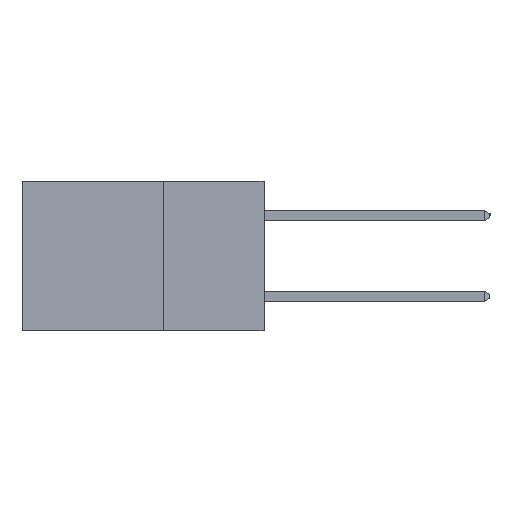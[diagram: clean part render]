
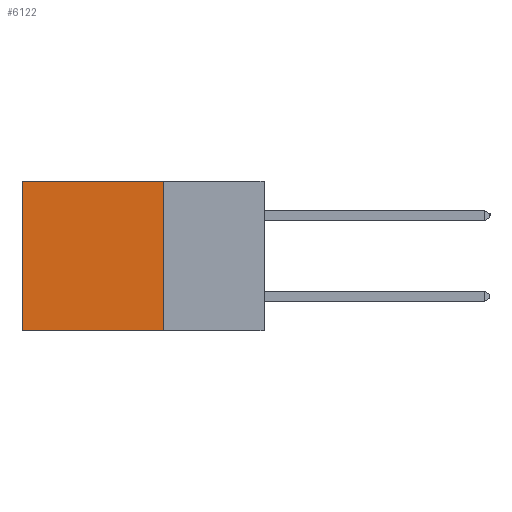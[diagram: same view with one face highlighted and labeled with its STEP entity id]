
A CAD part, left-side view. The second image highlights one B-rep face of the part: STEP entity #6122.
In plain terms, the highlighted planar face has unit normal (-1, 0, 0).
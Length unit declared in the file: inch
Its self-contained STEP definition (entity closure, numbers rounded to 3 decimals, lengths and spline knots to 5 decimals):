
#562 = AXIS2_PLACEMENT_3D ( 'NONE', #2618, #17270, #15629 ) ;
#961 = ORIENTED_EDGE ( 'NONE', *, *, #13653, .T. ) ;
#1107 = CARTESIAN_POINT ( 'NONE',  ( 0.2615, 0.6, -0.37 ) ) ;
#2184 = ORIENTED_EDGE ( 'NONE', *, *, #2893, .F. ) ;
#2618 = CARTESIAN_POINT ( 'NONE',  ( 0.2615, 0.25, -0.37 ) ) ;
#2893 = EDGE_CURVE ( 'NONE', #6404, #21108, #17577, .T. ) ;
#5316 = CARTESIAN_POINT ( 'NONE',  ( 0.2615, 0.6, 0. ) ) ;
#6122 = ADVANCED_FACE ( 'NONE', ( #20741 ), #10629, .F. ) ;
#6280 = LINE ( 'NONE', #11384, #17554 ) ;
#6404 = VERTEX_POINT ( 'NONE', #8318 ) ;
#6462 = VECTOR ( 'NONE', #18907, 39.37008 ) ;
#6482 = ORIENTED_EDGE ( 'NONE', *, *, #7011, .T. ) ;
#6521 = LINE ( 'NONE', #16502, #10236 ) ;
#6747 = EDGE_LOOP ( 'NONE', ( #961, #21380, #2184, #6482 ) ) ;
#7011 = EDGE_CURVE ( 'NONE', #6404, #10414, #6521, .T. ) ;
#7484 = VERTEX_POINT ( 'NONE', #17594 ) ;
#8318 = CARTESIAN_POINT ( 'NONE',  ( 0.2615, 0.25, 0. ) ) ;
#9434 = LINE ( 'NONE', #1107, #6462 ) ;
#9507 = CARTESIAN_POINT ( 'NONE',  ( 0.2615, 0.25, -0.37 ) ) ;
#9582 = CARTESIAN_POINT ( 'NONE',  ( 0.2615, 0.25, -0.37 ) ) ;
#10236 = VECTOR ( 'NONE', #21389, 39.37008 ) ;
#10414 = VERTEX_POINT ( 'NONE', #5316 ) ;
#10629 = PLANE ( 'NONE',  #562 ) ;
#11384 = CARTESIAN_POINT ( 'NONE',  ( 0.2615, 0.25, -0.37 ) ) ;
#13359 = VECTOR ( 'NONE', #16244, 39.37008 ) ;
#13653 = EDGE_CURVE ( 'NONE', #10414, #7484, #9434, .T. ) ;
#14375 = EDGE_CURVE ( 'NONE', #21108, #7484, #6280, .T. ) ;
#15629 = DIRECTION ( 'NONE',  ( 0., 0., -1. ) ) ;
#16244 = DIRECTION ( 'NONE',  ( 0., 0., -1. ) ) ;
#16502 = CARTESIAN_POINT ( 'NONE',  ( 0.2615, 0.25, 0. ) ) ;
#17270 = DIRECTION ( 'NONE',  ( 1., 0., 0. ) ) ;
#17554 = VECTOR ( 'NONE', #17792, 39.37008 ) ;
#17577 = LINE ( 'NONE', #9507, #13359 ) ;
#17594 = CARTESIAN_POINT ( 'NONE',  ( 0.2615, 0.6, -0.37 ) ) ;
#17792 = DIRECTION ( 'NONE',  ( 0., 1., 0. ) ) ;
#18907 = DIRECTION ( 'NONE',  ( 0., 0., -1. ) ) ;
#20741 = FACE_OUTER_BOUND ( 'NONE', #6747, .T. ) ;
#21108 = VERTEX_POINT ( 'NONE', #9582 ) ;
#21380 = ORIENTED_EDGE ( 'NONE', *, *, #14375, .F. ) ;
#21389 = DIRECTION ( 'NONE',  ( 0., 1., 0. ) ) ;
